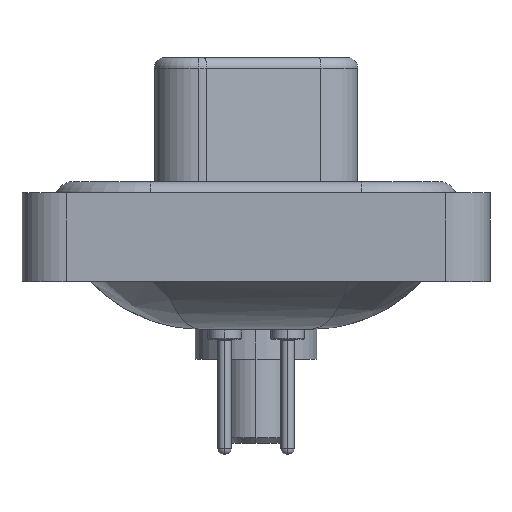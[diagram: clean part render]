
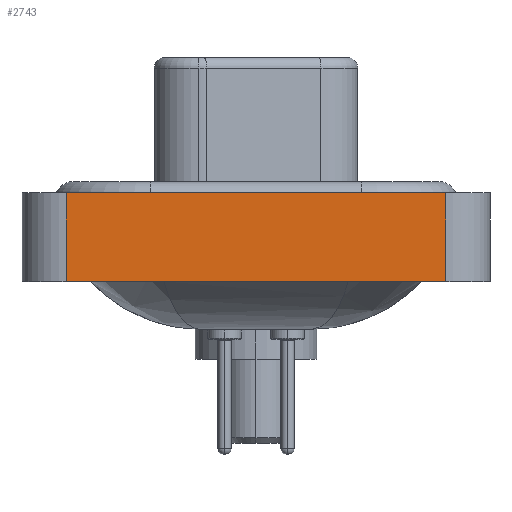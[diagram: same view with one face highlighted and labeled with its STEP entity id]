
A CAD part, left-side view. The second image highlights one B-rep face of the part: STEP entity #2743.
In plain terms, the highlighted planar face has unit normal (-1, 0, 0).
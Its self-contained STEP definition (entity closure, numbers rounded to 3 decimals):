
#857 = DIRECTION ( 'NONE',  ( 0., 0., 1. ) ) ;
#1085 = ORIENTED_EDGE ( 'NONE', *, *, #10281, .T. ) ;
#1149 = VERTEX_POINT ( 'NONE', #16589 ) ;
#1798 = LINE ( 'NONE', #9830, #6300 ) ;
#1854 = VERTEX_POINT ( 'NONE', #7762 ) ;
#2253 = AXIS2_PLACEMENT_3D ( 'NONE', #2376, #8875, #857 ) ;
#2376 = CARTESIAN_POINT ( 'NONE',  ( -7.25, -8.55, -3.6 ) ) ;
#2538 = CARTESIAN_POINT ( 'NONE',  ( -7.25, -8.55, -3.6 ) ) ;
#2743 = ADVANCED_FACE ( 'NONE', ( #3722 ), #11702, .T. ) ;
#3034 = EDGE_LOOP ( 'NONE', ( #11869, #5900, #7604, #1085 ) ) ;
#3722 = FACE_OUTER_BOUND ( 'NONE', #3034, .T. ) ;
#4286 = CARTESIAN_POINT ( 'NONE',  ( -7.25, 8.55, 0.4 ) ) ;
#4332 = LINE ( 'NONE', #9854, #9768 ) ;
#4509 = LINE ( 'NONE', #7490, #14209 ) ;
#4753 = EDGE_CURVE ( 'NONE', #5564, #6773, #4332, .T. ) ;
#5113 = EDGE_CURVE ( 'NONE', #1854, #5564, #1798, .T. ) ;
#5564 = VERTEX_POINT ( 'NONE', #4286 ) ;
#5789 = VECTOR ( 'NONE', #10691, 1000. ) ;
#5900 = ORIENTED_EDGE ( 'NONE', *, *, #4753, .F. ) ;
#6300 = VECTOR ( 'NONE', #12821, 1000. ) ;
#6773 = VERTEX_POINT ( 'NONE', #15434 ) ;
#7490 = CARTESIAN_POINT ( 'NONE',  ( -7.25, -8.55, -3.6 ) ) ;
#7557 = EDGE_CURVE ( 'NONE', #1149, #6773, #9222, .T. ) ;
#7604 = ORIENTED_EDGE ( 'NONE', *, *, #5113, .F. ) ;
#7762 = CARTESIAN_POINT ( 'NONE',  ( -7.25, 8.55, -3.6 ) ) ;
#8875 = DIRECTION ( 'NONE',  ( -1., 0., 0. ) ) ;
#9222 = LINE ( 'NONE', #2538, #5789 ) ;
#9768 = VECTOR ( 'NONE', #15382, 1000. ) ;
#9830 = CARTESIAN_POINT ( 'NONE',  ( -7.25, 8.55, -3.6 ) ) ;
#9854 = CARTESIAN_POINT ( 'NONE',  ( -7.25, -8.55, 0.4 ) ) ;
#10281 = EDGE_CURVE ( 'NONE', #1854, #1149, #4509, .T. ) ;
#10691 = DIRECTION ( 'NONE',  ( 0., 0., 1. ) ) ;
#11702 = PLANE ( 'NONE',  #2253 ) ;
#11869 = ORIENTED_EDGE ( 'NONE', *, *, #7557, .T. ) ;
#12821 = DIRECTION ( 'NONE',  ( 0., 0., 1. ) ) ;
#13020 = DIRECTION ( 'NONE',  ( 0., -1., 0. ) ) ;
#14209 = VECTOR ( 'NONE', #13020, 1000. ) ;
#15382 = DIRECTION ( 'NONE',  ( 0., -1., 0. ) ) ;
#15434 = CARTESIAN_POINT ( 'NONE',  ( -7.25, -8.55, 0.4 ) ) ;
#16589 = CARTESIAN_POINT ( 'NONE',  ( -7.25, -8.55, -3.6 ) ) ;
